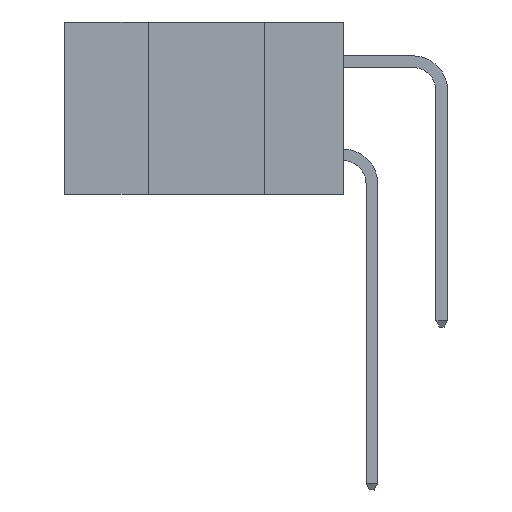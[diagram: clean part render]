
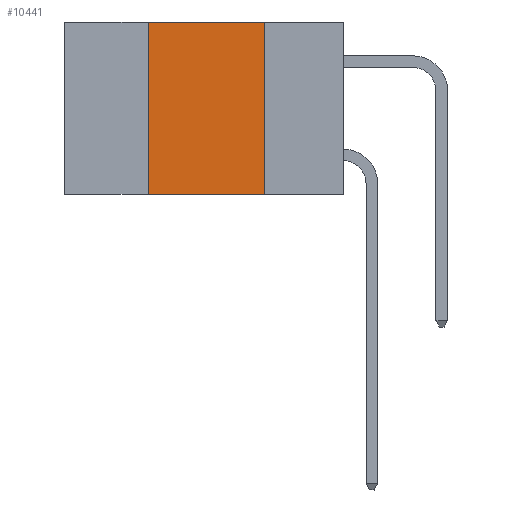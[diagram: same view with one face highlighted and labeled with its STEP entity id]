
A CAD part, left-side view. The second image highlights one B-rep face of the part: STEP entity #10441.
In plain terms, the highlighted planar face has unit normal (-1, 0, 0).
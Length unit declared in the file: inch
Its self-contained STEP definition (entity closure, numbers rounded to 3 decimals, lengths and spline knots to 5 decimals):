
#636 = LINE ( 'NONE', #14241, #22040 ) ;
#688 = EDGE_CURVE ( 'NONE', #25037, #26513, #13278, .T. ) ;
#1177 = DIRECTION ( 'NONE',  ( 0., -1., 0. ) ) ;
#1440 = VECTOR ( 'NONE', #1177, 39.37008 ) ;
#1578 = VECTOR ( 'NONE', #22191, 39.37008 ) ;
#2957 = VERTEX_POINT ( 'NONE', #11317 ) ;
#3615 = CARTESIAN_POINT ( 'NONE',  ( 0., 0.42, 0. ) ) ;
#5944 = PLANE ( 'NONE',  #14946 ) ;
#7664 = EDGE_CURVE ( 'NONE', #26513, #24883, #8190, .T. ) ;
#8190 = LINE ( 'NONE', #31421, #1578 ) ;
#8440 = DIRECTION ( 'NONE',  ( 0., 0., -1. ) ) ;
#9986 = EDGE_CURVE ( 'NONE', #2957, #25037, #636, .T. ) ;
#10441 = ADVANCED_FACE ( 'NONE', ( #25410 ), #5944, .F. ) ;
#11317 = CARTESIAN_POINT ( 'NONE',  ( 0., 0.42, -0.37 ) ) ;
#12478 = VECTOR ( 'NONE', #19959, 39.37008 ) ;
#12500 = CARTESIAN_POINT ( 'NONE',  ( 0., 0.6, 0. ) ) ;
#13125 = CARTESIAN_POINT ( 'NONE',  ( 0., 0.17, -0.37 ) ) ;
#13278 = LINE ( 'NONE', #12500, #12478 ) ;
#14241 = CARTESIAN_POINT ( 'NONE',  ( 0., 0.42, 0. ) ) ;
#14440 = ORIENTED_EDGE ( 'NONE', *, *, #9986, .F. ) ;
#14946 = AXIS2_PLACEMENT_3D ( 'NONE', #30488, #23311, #8440 ) ;
#16325 = ORIENTED_EDGE ( 'NONE', *, *, #21800, .T. ) ;
#17164 = EDGE_LOOP ( 'NONE', ( #23739, #19858, #14440, #16325 ) ) ;
#19858 = ORIENTED_EDGE ( 'NONE', *, *, #688, .F. ) ;
#19959 = DIRECTION ( 'NONE',  ( 0., -1., 0. ) ) ;
#21275 = LINE ( 'NONE', #30712, #1440 ) ;
#21800 = EDGE_CURVE ( 'NONE', #2957, #24883, #21275, .T. ) ;
#22040 = VECTOR ( 'NONE', #28944, 39.37008 ) ;
#22191 = DIRECTION ( 'NONE',  ( 0., 0., -1. ) ) ;
#23311 = DIRECTION ( 'NONE',  ( 1., 0., 0. ) ) ;
#23739 = ORIENTED_EDGE ( 'NONE', *, *, #7664, .F. ) ;
#24883 = VERTEX_POINT ( 'NONE', #13125 ) ;
#25037 = VERTEX_POINT ( 'NONE', #3615 ) ;
#25410 = FACE_OUTER_BOUND ( 'NONE', #17164, .T. ) ;
#26513 = VERTEX_POINT ( 'NONE', #28899 ) ;
#28899 = CARTESIAN_POINT ( 'NONE',  ( 0., 0.17, 0. ) ) ;
#28944 = DIRECTION ( 'NONE',  ( 0., 0., 1. ) ) ;
#30488 = CARTESIAN_POINT ( 'NONE',  ( 0., 0.6, 0. ) ) ;
#30712 = CARTESIAN_POINT ( 'NONE',  ( 0., 0.6, -0.37 ) ) ;
#31421 = CARTESIAN_POINT ( 'NONE',  ( 0., 0.17, 0. ) ) ;
